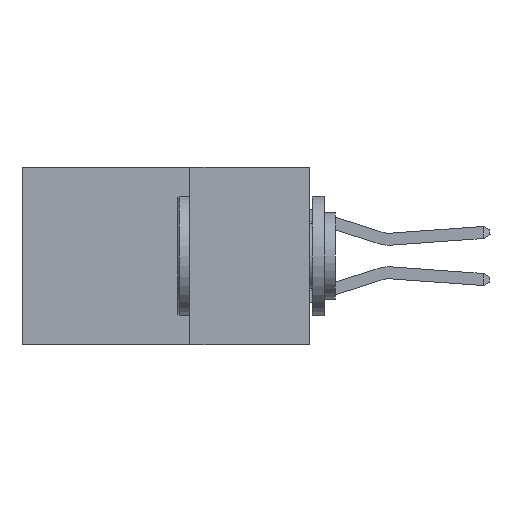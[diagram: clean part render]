
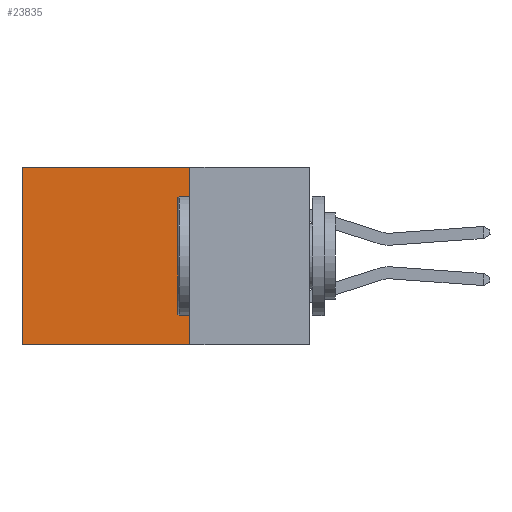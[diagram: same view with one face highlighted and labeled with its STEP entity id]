
A CAD part, left-side view. The second image highlights one B-rep face of the part: STEP entity #23835.
In plain terms, the highlighted planar face has unit normal (-1, 0, 0).
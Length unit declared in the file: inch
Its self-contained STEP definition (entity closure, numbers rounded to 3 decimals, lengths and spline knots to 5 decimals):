
#620 = FACE_OUTER_BOUND ( 'NONE', #21312, .T. ) ;
#1658 = ORIENTED_EDGE ( 'NONE', *, *, #6967, .F. ) ;
#1685 = CARTESIAN_POINT ( 'NONE',  ( 0.298, 0.25, -0.37 ) ) ;
#2501 = ORIENTED_EDGE ( 'NONE', *, *, #11331, .F. ) ;
#3041 = VECTOR ( 'NONE', #9087, 39.37008 ) ;
#3405 = CARTESIAN_POINT ( 'NONE',  ( 0.298, 0.6, -0.37 ) ) ;
#4468 = CARTESIAN_POINT ( 'NONE',  ( 0.298, 0.6, 0. ) ) ;
#5405 = VERTEX_POINT ( 'NONE', #4468 ) ;
#5910 = VECTOR ( 'NONE', #9862, 39.37008 ) ;
#5982 = CARTESIAN_POINT ( 'NONE',  ( 0.298, 0.25, 0. ) ) ;
#6210 = ORIENTED_EDGE ( 'NONE', *, *, #7422, .T. ) ;
#6967 = EDGE_CURVE ( 'NONE', #21409, #21812, #19241, .T. ) ;
#6978 = VECTOR ( 'NONE', #15380, 39.37008 ) ;
#7340 = CARTESIAN_POINT ( 'NONE',  ( 0.298, 0.25, 0. ) ) ;
#7422 = EDGE_CURVE ( 'NONE', #21409, #5405, #19214, .T. ) ;
#7800 = VECTOR ( 'NONE', #13484, 39.37008 ) ;
#8610 = ORIENTED_EDGE ( 'NONE', *, *, #15515, .T. ) ;
#9087 = DIRECTION ( 'NONE',  ( 0., 1., 0. ) ) ;
#9862 = DIRECTION ( 'NONE',  ( 0., 1., 0. ) ) ;
#10050 = DIRECTION ( 'NONE',  ( 1., 0., 0. ) ) ;
#11308 = LINE ( 'NONE', #1685, #5910 ) ;
#11313 = CARTESIAN_POINT ( 'NONE',  ( 0.298, 0.6, 0. ) ) ;
#11331 = EDGE_CURVE ( 'NONE', #21812, #13629, #11308, .T. ) ;
#12892 = AXIS2_PLACEMENT_3D ( 'NONE', #22191, #10050, #24212 ) ;
#13484 = DIRECTION ( 'NONE',  ( 0., 0., -1. ) ) ;
#13629 = VERTEX_POINT ( 'NONE', #3405 ) ;
#14032 = PLANE ( 'NONE',  #12892 ) ;
#15380 = DIRECTION ( 'NONE',  ( 0., 0., -1. ) ) ;
#15515 = EDGE_CURVE ( 'NONE', #5405, #13629, #17751, .T. ) ;
#17751 = LINE ( 'NONE', #11313, #6978 ) ;
#19214 = LINE ( 'NONE', #21246, #3041 ) ;
#19241 = LINE ( 'NONE', #7340, #7800 ) ;
#21246 = CARTESIAN_POINT ( 'NONE',  ( 0.298, 0.25, 0. ) ) ;
#21312 = EDGE_LOOP ( 'NONE', ( #8610, #2501, #1658, #6210 ) ) ;
#21409 = VERTEX_POINT ( 'NONE', #5982 ) ;
#21812 = VERTEX_POINT ( 'NONE', #25860 ) ;
#22191 = CARTESIAN_POINT ( 'NONE',  ( 0.298, 0.25, 0. ) ) ;
#23835 = ADVANCED_FACE ( 'NONE', ( #620 ), #14032, .F. ) ;
#24212 = DIRECTION ( 'NONE',  ( 0., 0., -1. ) ) ;
#25860 = CARTESIAN_POINT ( 'NONE',  ( 0.298, 0.25, -0.37 ) ) ;
